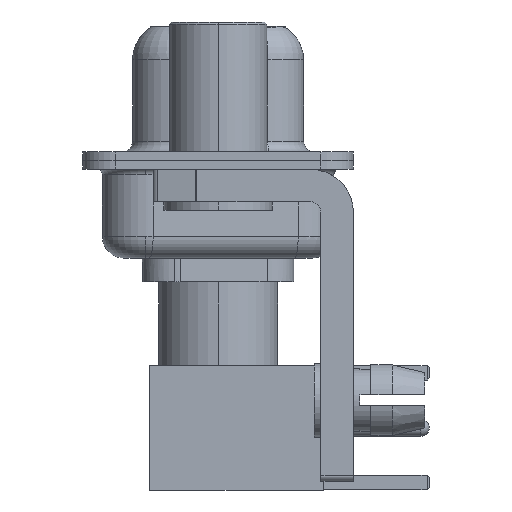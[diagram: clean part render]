
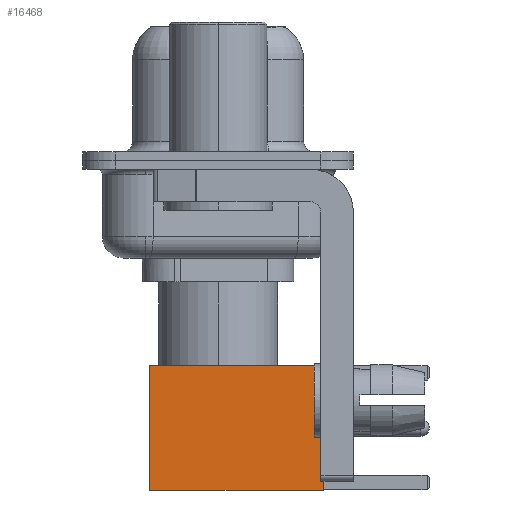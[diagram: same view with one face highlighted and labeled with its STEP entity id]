
A CAD part, left-side view. The second image highlights one B-rep face of the part: STEP entity #16468.
In plain terms, the highlighted face is planar.
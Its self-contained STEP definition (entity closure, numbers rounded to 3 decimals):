
#407 = VECTOR ( 'NONE', #8630, 1000. ) ;
#2855 = EDGE_CURVE ( 'NONE', #13148, #14978, #18059, .T. ) ;
#3040 = EDGE_CURVE ( 'NONE', #6340, #8962, #17455, .T. ) ;
#3260 = DIRECTION ( 'NONE',  ( 0., 1., 0. ) ) ;
#4333 = AXIS2_PLACEMENT_3D ( 'NONE', #6807, #3260, #18771 ) ;
#4415 = CARTESIAN_POINT ( 'NONE',  ( -2.875, 2.875, 0. ) ) ;
#4705 = LINE ( 'NONE', #9295, #17342 ) ;
#4792 = VECTOR ( 'NONE', #11682, 1000. ) ;
#4838 = CARTESIAN_POINT ( 'NONE',  ( 2.875, 2.875, 8. ) ) ;
#5422 = FACE_OUTER_BOUND ( 'NONE', #8110, .T. ) ;
#6340 = VERTEX_POINT ( 'NONE', #4838 ) ;
#6744 = ORIENTED_EDGE ( 'NONE', *, *, #2855, .F. ) ;
#6807 = CARTESIAN_POINT ( 'NONE',  ( 2.875, 2.875, 0. ) ) ;
#8110 = EDGE_LOOP ( 'NONE', ( #12091, #18116, #6744, #13886 ) ) ;
#8630 = DIRECTION ( 'NONE',  ( -1., 0., 0. ) ) ;
#8962 = VERTEX_POINT ( 'NONE', #19094 ) ;
#9295 = CARTESIAN_POINT ( 'NONE',  ( 0., 2.875, 0. ) ) ;
#10194 = CARTESIAN_POINT ( 'NONE',  ( 2.875, 2.875, 0. ) ) ;
#11682 = DIRECTION ( 'NONE',  ( 0., 0., -1. ) ) ;
#11858 = VECTOR ( 'NONE', #16566, 1000. ) ;
#12091 = ORIENTED_EDGE ( 'NONE', *, *, #3040, .T. ) ;
#12803 = CARTESIAN_POINT ( 'NONE',  ( -2.875, 2.875, 0. ) ) ;
#13148 = VERTEX_POINT ( 'NONE', #14808 ) ;
#13193 = EDGE_CURVE ( 'NONE', #6340, #13148, #14904, .T. ) ;
#13314 = CARTESIAN_POINT ( 'NONE',  ( 0., 2.875, 8. ) ) ;
#13886 = ORIENTED_EDGE ( 'NONE', *, *, #13193, .F. ) ;
#14502 = PLANE ( 'NONE',  #4333 ) ;
#14808 = CARTESIAN_POINT ( 'NONE',  ( -2.875, 2.875, 8. ) ) ;
#14904 = LINE ( 'NONE', #13314, #407 ) ;
#14978 = VERTEX_POINT ( 'NONE', #12803 ) ;
#15219 = EDGE_CURVE ( 'NONE', #8962, #14978, #4705, .T. ) ;
#16468 = ADVANCED_FACE ( 'NONE', ( #5422 ), #14502, .T. ) ;
#16566 = DIRECTION ( 'NONE',  ( 0., 0., -1. ) ) ;
#17342 = VECTOR ( 'NONE', #18247, 1000. ) ;
#17455 = LINE ( 'NONE', #10194, #4792 ) ;
#18059 = LINE ( 'NONE', #4415, #11858 ) ;
#18116 = ORIENTED_EDGE ( 'NONE', *, *, #15219, .T. ) ;
#18247 = DIRECTION ( 'NONE',  ( -1., 0., 0. ) ) ;
#18771 = DIRECTION ( 'NONE',  ( 0., 0., 1. ) ) ;
#19094 = CARTESIAN_POINT ( 'NONE',  ( 2.875, 2.875, 0. ) ) ;
